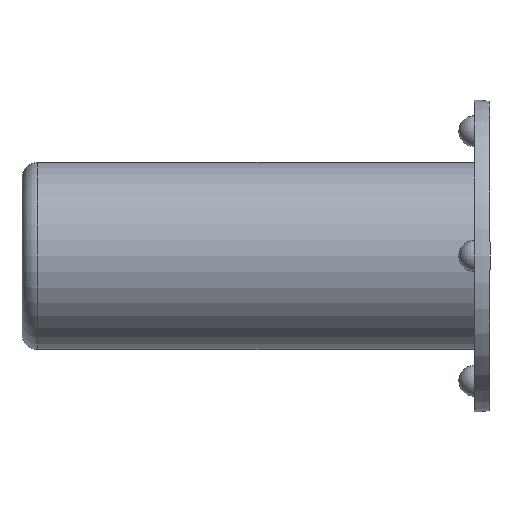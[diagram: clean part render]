
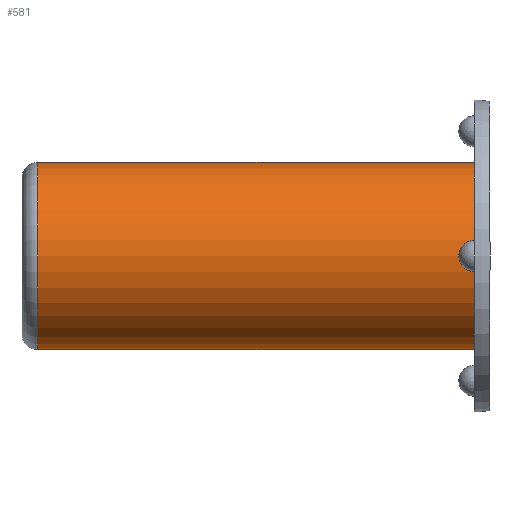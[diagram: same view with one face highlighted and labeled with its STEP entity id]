
A CAD part, left-side view. The second image highlights one B-rep face of the part: STEP entity #581.
In plain terms, the highlighted cylindrical face has radius 6 mm (diameter 12 mm), a full revolution.
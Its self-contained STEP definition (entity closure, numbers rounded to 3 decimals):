
#16 = CYLINDRICAL_SURFACE ( 'NONE', #768, 6. ) ;
#19 = FACE_OUTER_BOUND ( 'NONE', #1225, .T. ) ;
#48 = FACE_OUTER_BOUND ( 'NONE', #1214, .T. ) ;
#173 = VERTEX_POINT ( 'NONE', #579 ) ;
#186 = VERTEX_POINT ( 'NONE', #1309 ) ;
#207 = CARTESIAN_POINT ( 'NONE',  ( 0., 29., 0. ) ) ;
#288 = CARTESIAN_POINT ( 'NONE',  ( 0., 1., 0. ) ) ;
#302 = DIRECTION ( 'NONE',  ( 0., 0., 1. ) ) ;
#319 = AXIS2_PLACEMENT_3D ( 'NONE', #207, #948, #302 ) ;
#402 = DIRECTION ( 'NONE',  ( 0., 0., 1. ) ) ;
#570 = CIRCLE ( 'NONE', #319, 6. ) ;
#579 = CARTESIAN_POINT ( 'NONE',  ( 0., 29., 6. ) ) ;
#581 = ADVANCED_FACE ( 'NONE', ( #19, #48 ), #16, .T. ) ;
#614 = ORIENTED_EDGE ( 'NONE', *, *, #1175, .T. ) ;
#618 = CIRCLE ( 'NONE', #1198, 6. ) ;
#630 = ORIENTED_EDGE ( 'NONE', *, *, #1103, .F. ) ;
#650 = CARTESIAN_POINT ( 'NONE',  ( 0., 2., 0. ) ) ;
#761 = DIRECTION ( 'NONE',  ( 0., 0., -1. ) ) ;
#768 = AXIS2_PLACEMENT_3D ( 'NONE', #650, #961, #761 ) ;
#948 = DIRECTION ( 'NONE',  ( 0., -1., 0. ) ) ;
#961 = DIRECTION ( 'NONE',  ( 0., 1., 0. ) ) ;
#1036 = DIRECTION ( 'NONE',  ( 0., -1., 0. ) ) ;
#1103 = EDGE_CURVE ( 'NONE', #186, #186, #618, .T. ) ;
#1175 = EDGE_CURVE ( 'NONE', #173, #173, #570, .T. ) ;
#1198 = AXIS2_PLACEMENT_3D ( 'NONE', #288, #1036, #402 ) ;
#1214 = EDGE_LOOP ( 'NONE', ( #630 ) ) ;
#1225 = EDGE_LOOP ( 'NONE', ( #614 ) ) ;
#1309 = CARTESIAN_POINT ( 'NONE',  ( 0., 1., 6. ) ) ;
